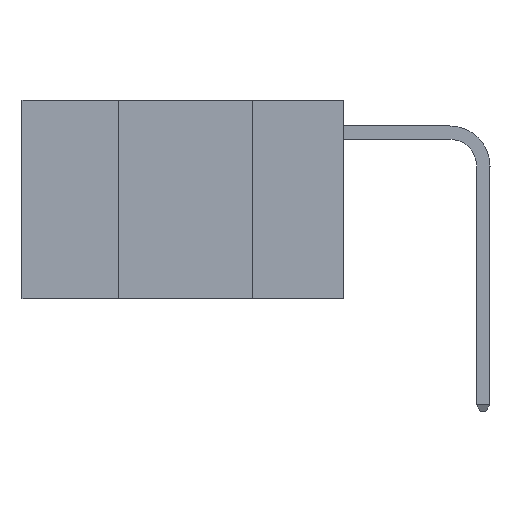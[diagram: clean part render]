
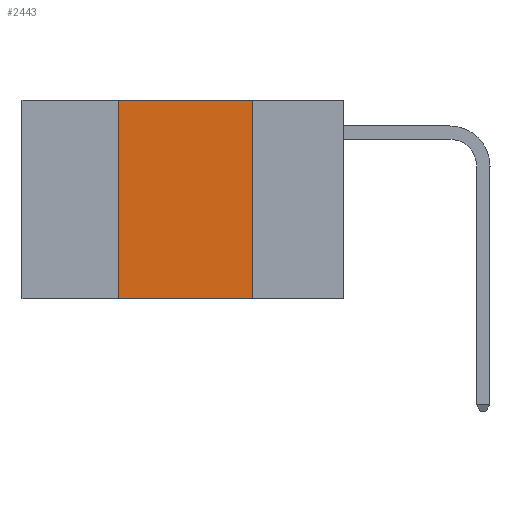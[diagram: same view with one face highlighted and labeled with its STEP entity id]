
A CAD part, left-side view. The second image highlights one B-rep face of the part: STEP entity #2443.
In plain terms, the highlighted planar face has unit normal (-1, 0, 0).
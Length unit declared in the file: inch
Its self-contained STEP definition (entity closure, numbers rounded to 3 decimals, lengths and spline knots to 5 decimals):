
#262 = AXIS2_PLACEMENT_3D ( 'NONE', #1685, #384, #1230 ) ;
#299 = ORIENTED_EDGE ( 'NONE', *, *, #1895, .F. ) ;
#384 = DIRECTION ( 'NONE',  ( 1., 0., 0. ) ) ;
#555 = CARTESIAN_POINT ( 'NONE',  ( 0., 0.42, -0.37 ) ) ;
#616 = VECTOR ( 'NONE', #762, 39.37008 ) ;
#739 = ORIENTED_EDGE ( 'NONE', *, *, #7381, .T. ) ;
#762 = DIRECTION ( 'NONE',  ( 0., 0., 1. ) ) ;
#1230 = DIRECTION ( 'NONE',  ( 0., 0., -1. ) ) ;
#1592 = CARTESIAN_POINT ( 'NONE',  ( 0., 0.17, -0.37 ) ) ;
#1685 = CARTESIAN_POINT ( 'NONE',  ( 0., 0.6, 0. ) ) ;
#1728 = PLANE ( 'NONE',  #262 ) ;
#1730 = VERTEX_POINT ( 'NONE', #1592 ) ;
#1895 = EDGE_CURVE ( 'NONE', #4324, #10238, #7606, .T. ) ;
#2443 = ADVANCED_FACE ( 'NONE', ( #12877 ), #1728, .F. ) ;
#3209 = CARTESIAN_POINT ( 'NONE',  ( 0., 0.17, 0. ) ) ;
#4284 = DIRECTION ( 'NONE',  ( 0., -1., 0. ) ) ;
#4324 = VERTEX_POINT ( 'NONE', #555 ) ;
#4346 = LINE ( 'NONE', #3209, #12696 ) ;
#5388 = CARTESIAN_POINT ( 'NONE',  ( 0., 0.42, 0. ) ) ;
#6150 = EDGE_LOOP ( 'NONE', ( #14347, #7284, #299, #739 ) ) ;
#6665 = VECTOR ( 'NONE', #14577, 39.37008 ) ;
#7054 = CARTESIAN_POINT ( 'NONE',  ( 0., 0.17, 0. ) ) ;
#7284 = ORIENTED_EDGE ( 'NONE', *, *, #7784, .F. ) ;
#7341 = DIRECTION ( 'NONE',  ( 0., 0., -1. ) ) ;
#7381 = EDGE_CURVE ( 'NONE', #4324, #1730, #10425, .T. ) ;
#7606 = LINE ( 'NONE', #5388, #616 ) ;
#7784 = EDGE_CURVE ( 'NONE', #10238, #17671, #15005, .T. ) ;
#10238 = VERTEX_POINT ( 'NONE', #17713 ) ;
#10425 = LINE ( 'NONE', #13140, #6665 ) ;
#11324 = CARTESIAN_POINT ( 'NONE',  ( 0., 0.6, 0. ) ) ;
#12386 = EDGE_CURVE ( 'NONE', #17671, #1730, #4346, .T. ) ;
#12696 = VECTOR ( 'NONE', #7341, 39.37008 ) ;
#12877 = FACE_OUTER_BOUND ( 'NONE', #6150, .T. ) ;
#13140 = CARTESIAN_POINT ( 'NONE',  ( 0., 0.6, -0.37 ) ) ;
#14347 = ORIENTED_EDGE ( 'NONE', *, *, #12386, .F. ) ;
#14577 = DIRECTION ( 'NONE',  ( 0., -1., 0. ) ) ;
#14580 = VECTOR ( 'NONE', #4284, 39.37008 ) ;
#15005 = LINE ( 'NONE', #11324, #14580 ) ;
#17671 = VERTEX_POINT ( 'NONE', #7054 ) ;
#17713 = CARTESIAN_POINT ( 'NONE',  ( 0., 0.42, 0. ) ) ;
